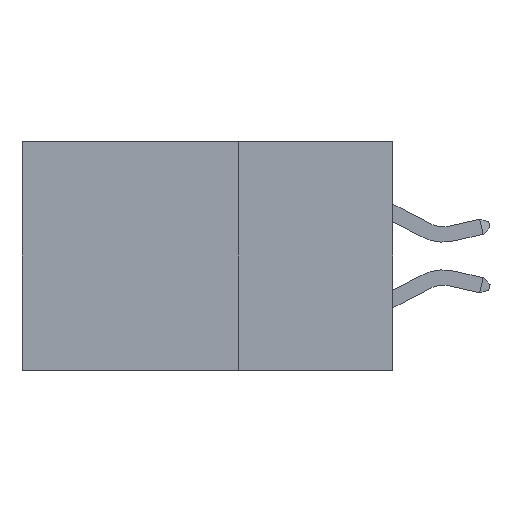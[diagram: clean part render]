
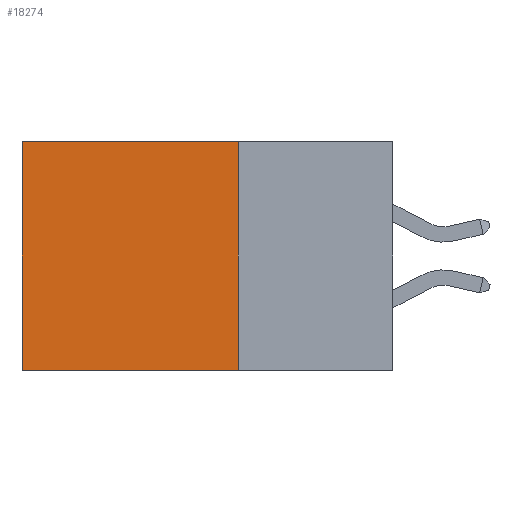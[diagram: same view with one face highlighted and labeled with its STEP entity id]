
A CAD part, left-side view. The second image highlights one B-rep face of the part: STEP entity #18274.
In plain terms, the highlighted planar face has unit normal (-1, 0, 0).
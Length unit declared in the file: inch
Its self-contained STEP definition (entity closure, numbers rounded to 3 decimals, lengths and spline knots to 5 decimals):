
#238 = CARTESIAN_POINT ( 'NONE',  ( 0.2875, 0.25, -0.37 ) ) ;
#582 = VERTEX_POINT ( 'NONE', #12229 ) ;
#656 = ORIENTED_EDGE ( 'NONE', *, *, #18414, .T. ) ;
#917 = CARTESIAN_POINT ( 'NONE',  ( 0.2875, 0.6, -0.37 ) ) ;
#1961 = DIRECTION ( 'NONE',  ( 0., 1., 0. ) ) ;
#2061 = VERTEX_POINT ( 'NONE', #4880 ) ;
#2353 = CARTESIAN_POINT ( 'NONE',  ( 0.2875, 0.25, 0. ) ) ;
#3597 = VECTOR ( 'NONE', #1961, 39.37008 ) ;
#4262 = ORIENTED_EDGE ( 'NONE', *, *, #17590, .F. ) ;
#4451 = ORIENTED_EDGE ( 'NONE', *, *, #16965, .F. ) ;
#4870 = CARTESIAN_POINT ( 'NONE',  ( 0.2875, 0.25, -0.37 ) ) ;
#4880 = CARTESIAN_POINT ( 'NONE',  ( 0.2875, 0.25, 0. ) ) ;
#5770 = DIRECTION ( 'NONE',  ( 0., 0., -1. ) ) ;
#6564 = DIRECTION ( 'NONE',  ( 0., 1., 0. ) ) ;
#6793 = LINE ( 'NONE', #8867, #18324 ) ;
#6991 = PLANE ( 'NONE',  #19048 ) ;
#8347 = VERTEX_POINT ( 'NONE', #4870 ) ;
#8798 = CARTESIAN_POINT ( 'NONE',  ( 0.2875, 0.25, 0. ) ) ;
#8867 = CARTESIAN_POINT ( 'NONE',  ( 0.2875, 0.6, 0. ) ) ;
#9821 = LINE ( 'NONE', #238, #3597 ) ;
#12229 = CARTESIAN_POINT ( 'NONE',  ( 0.2875, 0.6, 0. ) ) ;
#13460 = VERTEX_POINT ( 'NONE', #917 ) ;
#13602 = VECTOR ( 'NONE', #16944, 39.37008 ) ;
#13696 = EDGE_CURVE ( 'NONE', #2061, #582, #14522, .T. ) ;
#14408 = CARTESIAN_POINT ( 'NONE',  ( 0.2875, 0.25, 0. ) ) ;
#14522 = LINE ( 'NONE', #14408, #17063 ) ;
#16030 = EDGE_LOOP ( 'NONE', ( #656, #4262, #4451, #16391 ) ) ;
#16391 = ORIENTED_EDGE ( 'NONE', *, *, #13696, .T. ) ;
#16794 = DIRECTION ( 'NONE',  ( 0., 0., -1. ) ) ;
#16944 = DIRECTION ( 'NONE',  ( 0., 0., -1. ) ) ;
#16965 = EDGE_CURVE ( 'NONE', #2061, #8347, #18120, .T. ) ;
#17063 = VECTOR ( 'NONE', #6564, 39.37008 ) ;
#17590 = EDGE_CURVE ( 'NONE', #8347, #13460, #9821, .T. ) ;
#18120 = LINE ( 'NONE', #2353, #13602 ) ;
#18274 = ADVANCED_FACE ( 'NONE', ( #19599 ), #6991, .F. ) ;
#18324 = VECTOR ( 'NONE', #5770, 39.37008 ) ;
#18414 = EDGE_CURVE ( 'NONE', #582, #13460, #6793, .T. ) ;
#19048 = AXIS2_PLACEMENT_3D ( 'NONE', #8798, #19786, #16794 ) ;
#19599 = FACE_OUTER_BOUND ( 'NONE', #16030, .T. ) ;
#19786 = DIRECTION ( 'NONE',  ( 1., 0., 0. ) ) ;
